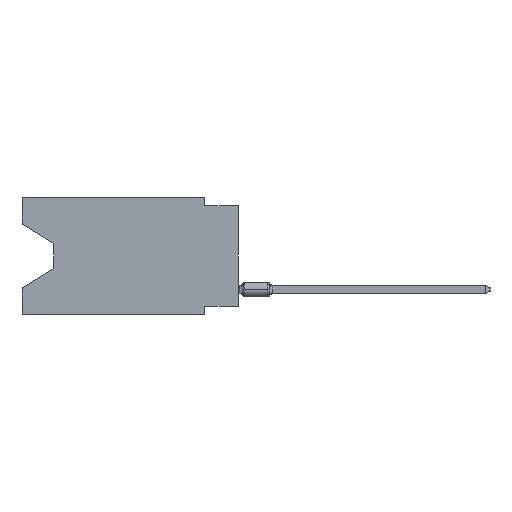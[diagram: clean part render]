
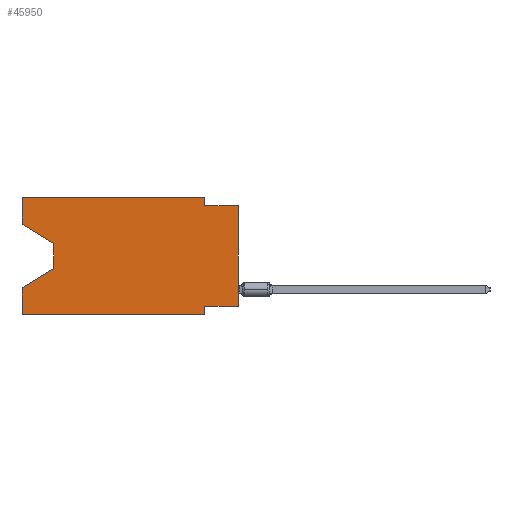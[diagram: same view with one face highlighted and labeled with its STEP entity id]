
A CAD part, left-side view. The second image highlights one B-rep face of the part: STEP entity #45950.
In plain terms, the highlighted planar face has unit normal (-1, 0, 0).
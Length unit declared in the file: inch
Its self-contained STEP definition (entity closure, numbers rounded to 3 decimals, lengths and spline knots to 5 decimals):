
#372 = DIRECTION ( 'NONE',  ( 0., 0.855, -0.519 ) ) ;
#449 = VERTEX_POINT ( 'NONE', #9278 ) ;
#1099 = CARTESIAN_POINT ( 'NONE',  ( 0., 0., -0.025 ) ) ;
#2227 = LINE ( 'NONE', #17350, #58523 ) ;
#2698 = VECTOR ( 'NONE', #11333, 39.37008 ) ;
#6787 = LINE ( 'NONE', #7131, #25916 ) ;
#7131 = CARTESIAN_POINT ( 'NONE',  ( 0., 0.645, 0. ) ) ;
#8281 = VERTEX_POINT ( 'NONE', #59858 ) ;
#8596 = VECTOR ( 'NONE', #52292, 39.37008 ) ;
#8799 = EDGE_CURVE ( 'NONE', #27529, #15963, #57540, .T. ) ;
#9136 = DIRECTION ( 'NONE',  ( 0., 0., 1. ) ) ;
#9278 = CARTESIAN_POINT ( 'NONE',  ( 0., 0.1, 0. ) ) ;
#9743 = EDGE_CURVE ( 'NONE', #28734, #8281, #6787, .T. ) ;
#10024 = LINE ( 'NONE', #37754, #29495 ) ;
#10349 = ORIENTED_EDGE ( 'NONE', *, *, #28203, .F. ) ;
#10737 = CARTESIAN_POINT ( 'NONE',  ( 0., 0.645, -0.26975 ) ) ;
#10826 = CARTESIAN_POINT ( 'NONE',  ( 0., 0.1, -0.35 ) ) ;
#11042 = EDGE_CURVE ( 'NONE', #59823, #61893, #2227, .T. ) ;
#11333 = DIRECTION ( 'NONE',  ( 0., 0., -1. ) ) ;
#13095 = ORIENTED_EDGE ( 'NONE', *, *, #11042, .F. ) ;
#13205 = VERTEX_POINT ( 'NONE', #1099 ) ;
#13388 = VERTEX_POINT ( 'NONE', #42395 ) ;
#13866 = CARTESIAN_POINT ( 'NONE',  ( 0., 0.1, -0.35 ) ) ;
#15277 = VECTOR ( 'NONE', #9136, 39.37008 ) ;
#15815 = LINE ( 'NONE', #64236, #53471 ) ;
#15963 = VERTEX_POINT ( 'NONE', #32644 ) ;
#16538 = ORIENTED_EDGE ( 'NONE', *, *, #58831, .F. ) ;
#17350 = CARTESIAN_POINT ( 'NONE',  ( 0., 0.645, 0. ) ) ;
#17795 = EDGE_CURVE ( 'NONE', #68706, #13388, #49173, .T. ) ;
#20705 = VERTEX_POINT ( 'NONE', #64670 ) ;
#20856 = CARTESIAN_POINT ( 'NONE',  ( 0., 0.1, 0. ) ) ;
#20906 = ORIENTED_EDGE ( 'NONE', *, *, #8799, .T. ) ;
#21712 = DIRECTION ( 'NONE',  ( 1., 0., 0. ) ) ;
#21960 = DIRECTION ( 'NONE',  ( 0., -1., 0. ) ) ;
#22378 = EDGE_LOOP ( 'NONE', ( #58880, #20906, #44817, #13095, #46487, #40388, #61336, #29352, #32495, #10349, #16538, #69396 ) ) ;
#23545 = LINE ( 'NONE', #44964, #39009 ) ;
#24925 = DIRECTION ( 'NONE',  ( 0., -1., 0. ) ) ;
#25916 = VECTOR ( 'NONE', #60819, 39.37008 ) ;
#27529 = VERTEX_POINT ( 'NONE', #42015 ) ;
#27980 = VERTEX_POINT ( 'NONE', #13866 ) ;
#28203 = EDGE_CURVE ( 'NONE', #449, #20705, #42625, .T. ) ;
#28734 = VERTEX_POINT ( 'NONE', #33019 ) ;
#29352 = ORIENTED_EDGE ( 'NONE', *, *, #32663, .T. ) ;
#29495 = VECTOR ( 'NONE', #21960, 39.37008 ) ;
#30881 = CARTESIAN_POINT ( 'NONE',  ( 0., 0., -0.325 ) ) ;
#32493 = LINE ( 'NONE', #64768, #36170 ) ;
#32495 = ORIENTED_EDGE ( 'NONE', *, *, #50564, .F. ) ;
#32644 = CARTESIAN_POINT ( 'NONE',  ( 0., 0.55, -0.212 ) ) ;
#32663 = EDGE_CURVE ( 'NONE', #68706, #13205, #63513, .T. ) ;
#33019 = CARTESIAN_POINT ( 'NONE',  ( 0., 0.645, -0.08025 ) ) ;
#33234 = AXIS2_PLACEMENT_3D ( 'NONE', #64851, #21712, #42780 ) ;
#34864 = DIRECTION ( 'NONE',  ( 0., 0., 1. ) ) ;
#35353 = LINE ( 'NONE', #56754, #50758 ) ;
#35375 = EDGE_CURVE ( 'NONE', #13388, #27980, #58916, .T. ) ;
#36128 = FACE_OUTER_BOUND ( 'NONE', #22378, .T. ) ;
#36170 = VECTOR ( 'NONE', #54255, 39.37008 ) ;
#37740 = VECTOR ( 'NONE', #68998, 39.37008 ) ;
#37754 = CARTESIAN_POINT ( 'NONE',  ( 0., 0.645, 0. ) ) ;
#39009 = VECTOR ( 'NONE', #24925, 39.37008 ) ;
#39511 = EDGE_CURVE ( 'NONE', #59823, #27980, #35353, .T. ) ;
#39808 = EDGE_CURVE ( 'NONE', #28734, #27529, #32493, .T. ) ;
#39933 = DIRECTION ( 'NONE',  ( 0., -1., 0. ) ) ;
#40388 = ORIENTED_EDGE ( 'NONE', *, *, #35375, .F. ) ;
#42015 = CARTESIAN_POINT ( 'NONE',  ( 0., 0.55, -0.138 ) ) ;
#42395 = CARTESIAN_POINT ( 'NONE',  ( 0., 0.1, -0.325 ) ) ;
#42625 = LINE ( 'NONE', #20856, #2698 ) ;
#42780 = DIRECTION ( 'NONE',  ( 0., 0., -1. ) ) ;
#43139 = DIRECTION ( 'NONE',  ( 0., 0., -1. ) ) ;
#44817 = ORIENTED_EDGE ( 'NONE', *, *, #64679, .T. ) ;
#44964 = CARTESIAN_POINT ( 'NONE',  ( 0., 0., -0.025 ) ) ;
#45950 = ADVANCED_FACE ( 'NONE', ( #36128 ), #57522, .F. ) ;
#46487 = ORIENTED_EDGE ( 'NONE', *, *, #39511, .T. ) ;
#49173 = LINE ( 'NONE', #63734, #37740 ) ;
#50564 = EDGE_CURVE ( 'NONE', #20705, #13205, #23545, .T. ) ;
#50758 = VECTOR ( 'NONE', #39933, 39.37008 ) ;
#52292 = DIRECTION ( 'NONE',  ( 0., 0., -1. ) ) ;
#53471 = VECTOR ( 'NONE', #372, 39.37008 ) ;
#54255 = DIRECTION ( 'NONE',  ( 0., -0.855, -0.519 ) ) ;
#56754 = CARTESIAN_POINT ( 'NONE',  ( 0., 0.645, -0.35 ) ) ;
#57221 = CARTESIAN_POINT ( 'NONE',  ( 0., 0., 0. ) ) ;
#57522 = PLANE ( 'NONE',  #33234 ) ;
#57540 = LINE ( 'NONE', #67721, #8596 ) ;
#58137 = VECTOR ( 'NONE', #43139, 39.37008 ) ;
#58287 = CARTESIAN_POINT ( 'NONE',  ( 0., 0.645, -0.35 ) ) ;
#58523 = VECTOR ( 'NONE', #34864, 39.37008 ) ;
#58831 = EDGE_CURVE ( 'NONE', #8281, #449, #10024, .T. ) ;
#58880 = ORIENTED_EDGE ( 'NONE', *, *, #39808, .T. ) ;
#58916 = LINE ( 'NONE', #10826, #58137 ) ;
#59823 = VERTEX_POINT ( 'NONE', #58287 ) ;
#59858 = CARTESIAN_POINT ( 'NONE',  ( 0., 0.645, 0. ) ) ;
#60819 = DIRECTION ( 'NONE',  ( 0., 0., 1. ) ) ;
#61336 = ORIENTED_EDGE ( 'NONE', *, *, #17795, .F. ) ;
#61893 = VERTEX_POINT ( 'NONE', #10737 ) ;
#63513 = LINE ( 'NONE', #57221, #15277 ) ;
#63734 = CARTESIAN_POINT ( 'NONE',  ( 0., 0., -0.325 ) ) ;
#64236 = CARTESIAN_POINT ( 'NONE',  ( 0., 0.55, -0.212 ) ) ;
#64670 = CARTESIAN_POINT ( 'NONE',  ( 0., 0.1, -0.025 ) ) ;
#64679 = EDGE_CURVE ( 'NONE', #15963, #61893, #15815, .T. ) ;
#64768 = CARTESIAN_POINT ( 'NONE',  ( 0., 0.645, -0.08025 ) ) ;
#64851 = CARTESIAN_POINT ( 'NONE',  ( 0., 0.645, 0. ) ) ;
#67721 = CARTESIAN_POINT ( 'NONE',  ( 0., 0.55, -0.138 ) ) ;
#68706 = VERTEX_POINT ( 'NONE', #30881 ) ;
#68998 = DIRECTION ( 'NONE',  ( 0., 1., 0. ) ) ;
#69396 = ORIENTED_EDGE ( 'NONE', *, *, #9743, .F. ) ;
